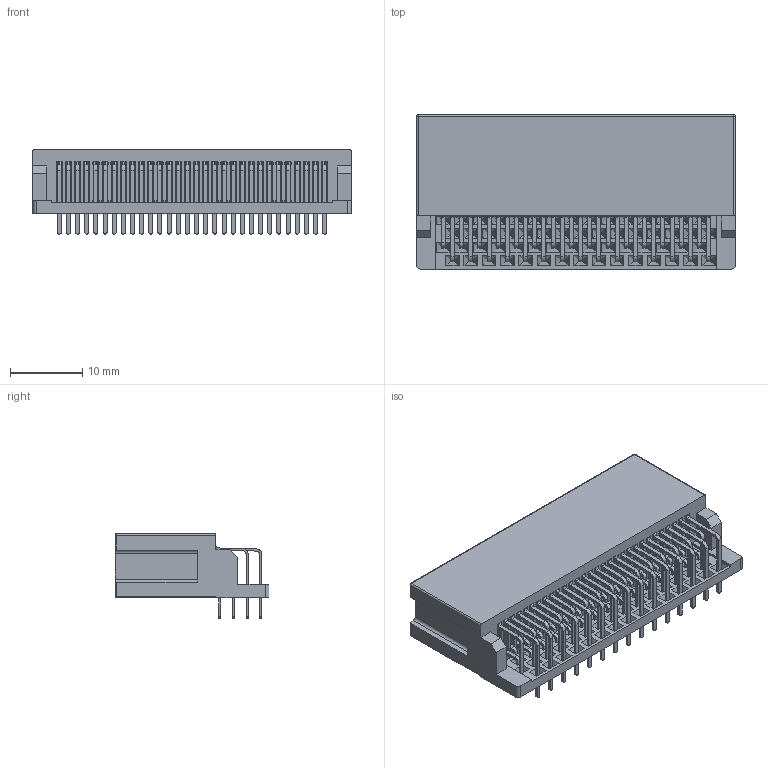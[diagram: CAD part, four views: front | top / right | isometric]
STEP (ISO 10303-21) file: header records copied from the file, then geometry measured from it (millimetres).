
FILE_DESCRIPTION (( 'STEP AP203' ), '1' );
FILE_NAME ('302-060-658-201.STEP', '2024-04-01T21:54:57', ( '' ), ( '' ), 'SwSTEP 2.0', 'SolidWorks 2023', '' );
FILE_SCHEMA (( 'CONFIG_CONTROL_DESIGN' ));
Length unit declared in the file: millimetre
Products named in the file (6): 302-060-658-201; Contact_302-290-X58-003; Contact_302-290-X58-001; HSG_RA HSG; Contact_302-290-X58-002; Contact_302-290-X58-004
Assembly tree (61 placements, depth 2):
  302-060-658-201
    HSG_RA HSG
    Contact_302-290-X58-003  x15
    Contact_302-290-X58-004  x15
    Contact_302-290-X58-001  x15
    Contact_302-290-X58-002  x15
Bounding box: 44.2 x 21.37 x 11.68 mm (x, y, z)
Volume: 3969.6 mm3; surface area: 10861.8 mm2
Topology: 61 solids, 61 shells, 3181 faces, 9519 edges, 6278 vertices
Faces by surface type: plane 2263, cylinder 794, bspline 120, sphere 4
Entity records: 37670 total; most frequent: CARTESIAN_POINT 7029, ORIENTED_EDGE 6486, DIRECTION 5172, EDGE_CURVE 3243, VECTOR 2914, LINE 2914, VERTEX_POINT 2134, AXIS2_PLACEMENT_3D 1129
